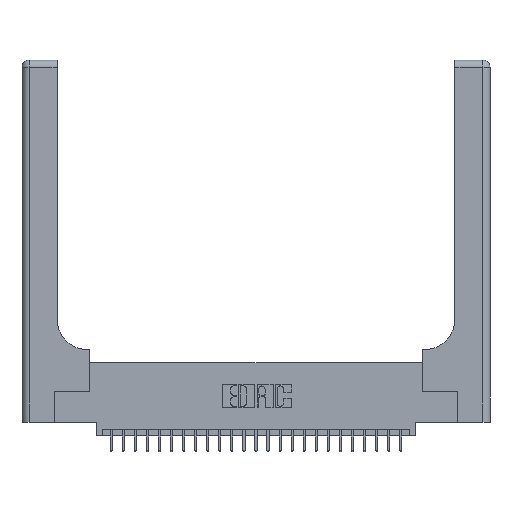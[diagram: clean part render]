
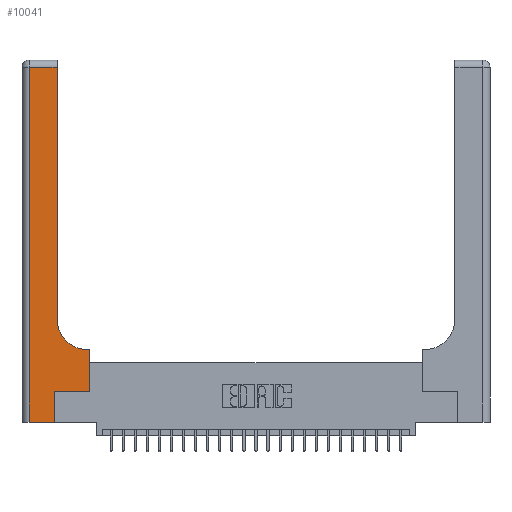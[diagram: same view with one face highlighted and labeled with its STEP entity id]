
A CAD part, top view. The second image highlights one B-rep face of the part: STEP entity #10041.
In plain terms, the highlighted planar face has unit normal (0, 0, 1).
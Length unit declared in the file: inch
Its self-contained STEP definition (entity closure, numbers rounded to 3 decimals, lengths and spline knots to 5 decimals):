
#412 = CARTESIAN_POINT ( 'NONE',  ( 0., 0., 0.37 ) ) ;
#465 = EDGE_CURVE ( 'NONE', #20732, #14692, #9370, .T. ) ;
#664 = LINE ( 'NONE', #7572, #19293 ) ;
#746 = EDGE_LOOP ( 'NONE', ( #26284, #5387, #11602, #6184, #8859, #12666, #22089, #15127, #2855 ) ) ;
#942 = DIRECTION ( 'NONE',  ( 1., 0., 0. ) ) ;
#1602 = VECTOR ( 'NONE', #11873, 39.37008 ) ;
#2000 = PLANE ( 'NONE',  #16144 ) ;
#2007 = VECTOR ( 'NONE', #3231, 39.37008 ) ;
#2326 = VECTOR ( 'NONE', #6742, 39.37008 ) ;
#2676 = CARTESIAN_POINT ( 'NONE',  ( 0.06, 3., 0.37 ) ) ;
#2855 = ORIENTED_EDGE ( 'NONE', *, *, #6508, .T. ) ;
#3231 = DIRECTION ( 'NONE',  ( -1., 0., 0. ) ) ;
#3444 = CARTESIAN_POINT ( 'NONE',  ( 0.269, 0., 0.37 ) ) ;
#3466 = LINE ( 'NONE', #15884, #11018 ) ;
#4506 = DIRECTION ( 'NONE',  ( 0., 0., -1. ) ) ;
#5310 = LINE ( 'NONE', #9598, #2007 ) ;
#5320 = EDGE_CURVE ( 'NONE', #20075, #20732, #26034, .T. ) ;
#5387 = ORIENTED_EDGE ( 'NONE', *, *, #23144, .T. ) ;
#5877 = AXIS2_PLACEMENT_3D ( 'NONE', #17088, #4506, #23591 ) ;
#6110 = CARTESIAN_POINT ( 'NONE',  ( 0.2915, 2.94, 0.37 ) ) ;
#6123 = EDGE_CURVE ( 'NONE', #25892, #10410, #24753, .T. ) ;
#6184 = ORIENTED_EDGE ( 'NONE', *, *, #465, .T. ) ;
#6508 = EDGE_CURVE ( 'NONE', #11296, #25892, #21767, .T. ) ;
#6677 = DIRECTION ( 'NONE',  ( 0., -1., 0. ) ) ;
#6742 = DIRECTION ( 'NONE',  ( 0., 1., 0. ) ) ;
#6872 = VECTOR ( 'NONE', #942, 39.37008 ) ;
#7572 = CARTESIAN_POINT ( 'NONE',  ( 0.269, 0.25, 0.37 ) ) ;
#8484 = FACE_OUTER_BOUND ( 'NONE', #746, .T. ) ;
#8859 = ORIENTED_EDGE ( 'NONE', *, *, #26110, .T. ) ;
#9370 = LINE ( 'NONE', #412, #6872 ) ;
#9551 = EDGE_CURVE ( 'NONE', #19928, #24577, #22929, .T. ) ;
#9598 = CARTESIAN_POINT ( 'NONE',  ( 0., 2.94, 0.37 ) ) ;
#10041 = ADVANCED_FACE ( 'NONE', ( #8484 ), #2000, .F. ) ;
#10410 = VERTEX_POINT ( 'NONE', #6110 ) ;
#11018 = VECTOR ( 'NONE', #26830, 39.37008 ) ;
#11046 = CARTESIAN_POINT ( 'NONE',  ( 0.269, 0., 0.37 ) ) ;
#11151 = CARTESIAN_POINT ( 'NONE',  ( 0.5585, 0.25, 0.37 ) ) ;
#11296 = VERTEX_POINT ( 'NONE', #25237 ) ;
#11300 = DIRECTION ( 'NONE',  ( 1., 0., 0. ) ) ;
#11602 = ORIENTED_EDGE ( 'NONE', *, *, #5320, .T. ) ;
#11873 = DIRECTION ( 'NONE',  ( 0., 1., 0. ) ) ;
#12666 = ORIENTED_EDGE ( 'NONE', *, *, #12915, .T. ) ;
#12703 = VERTEX_POINT ( 'NONE', #16327 ) ;
#12915 = EDGE_CURVE ( 'NONE', #12703, #19928, #664, .T. ) ;
#13255 = CARTESIAN_POINT ( 'NONE',  ( 0.2915, 3., 0.37 ) ) ;
#14692 = VERTEX_POINT ( 'NONE', #11046 ) ;
#15127 = ORIENTED_EDGE ( 'NONE', *, *, #15739, .T. ) ;
#15182 = CARTESIAN_POINT ( 'NONE',  ( 0.2915, 0.85, 0.37 ) ) ;
#15739 = EDGE_CURVE ( 'NONE', #24577, #11296, #3466, .T. ) ;
#15884 = CARTESIAN_POINT ( 'NONE',  ( 0.2915, 0.6, 0.37 ) ) ;
#16144 = AXIS2_PLACEMENT_3D ( 'NONE', #18583, #25235, #27037 ) ;
#16327 = CARTESIAN_POINT ( 'NONE',  ( 0.269, 0.25, 0.37 ) ) ;
#17088 = CARTESIAN_POINT ( 'NONE',  ( 0.5415, 0.85, 0.37 ) ) ;
#18583 = CARTESIAN_POINT ( 'NONE',  ( 0., 3., 0.37 ) ) ;
#19062 = CARTESIAN_POINT ( 'NONE',  ( 0.5585, 0.6, 0.37 ) ) ;
#19293 = VECTOR ( 'NONE', #11300, 39.37008 ) ;
#19928 = VERTEX_POINT ( 'NONE', #11151 ) ;
#19977 = CARTESIAN_POINT ( 'NONE',  ( 0.06, 2.94, 0.37 ) ) ;
#20075 = VERTEX_POINT ( 'NONE', #19977 ) ;
#20732 = VERTEX_POINT ( 'NONE', #22312 ) ;
#21115 = DIRECTION ( 'NONE',  ( 0., 1., 0. ) ) ;
#21767 = CIRCLE ( 'NONE', #5877, 0.25 ) ;
#22089 = ORIENTED_EDGE ( 'NONE', *, *, #9551, .T. ) ;
#22242 = LINE ( 'NONE', #3444, #1602 ) ;
#22312 = CARTESIAN_POINT ( 'NONE',  ( 0.06, 0., 0.37 ) ) ;
#22929 = LINE ( 'NONE', #23192, #24081 ) ;
#23144 = EDGE_CURVE ( 'NONE', #10410, #20075, #5310, .T. ) ;
#23192 = CARTESIAN_POINT ( 'NONE',  ( 0.5585, 0.25, 0.37 ) ) ;
#23509 = VECTOR ( 'NONE', #6677, 39.37008 ) ;
#23591 = DIRECTION ( 'NONE',  ( 1., 0., 0. ) ) ;
#24081 = VECTOR ( 'NONE', #21115, 39.37008 ) ;
#24577 = VERTEX_POINT ( 'NONE', #19062 ) ;
#24753 = LINE ( 'NONE', #13255, #2326 ) ;
#25235 = DIRECTION ( 'NONE',  ( 0., 0., -1. ) ) ;
#25237 = CARTESIAN_POINT ( 'NONE',  ( 0.5415, 0.6, 0.37 ) ) ;
#25892 = VERTEX_POINT ( 'NONE', #15182 ) ;
#26034 = LINE ( 'NONE', #2676, #23509 ) ;
#26110 = EDGE_CURVE ( 'NONE', #14692, #12703, #22242, .T. ) ;
#26284 = ORIENTED_EDGE ( 'NONE', *, *, #6123, .T. ) ;
#26830 = DIRECTION ( 'NONE',  ( -1., 0., 0. ) ) ;
#27037 = DIRECTION ( 'NONE',  ( -1., 0., 0. ) ) ;
